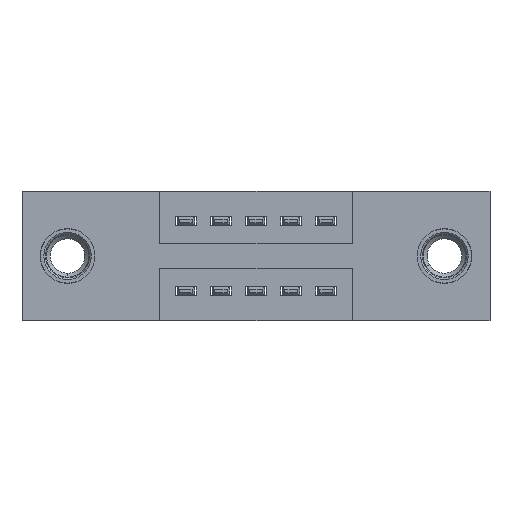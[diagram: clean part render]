
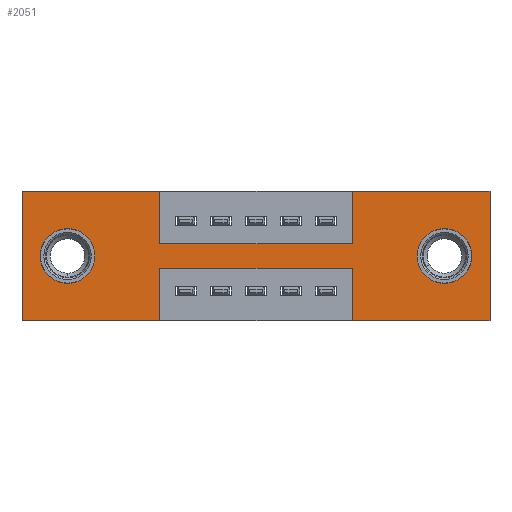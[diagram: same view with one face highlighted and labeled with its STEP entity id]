
A CAD part, front view. The second image highlights one B-rep face of the part: STEP entity #2051.
In plain terms, the highlighted planar face has unit normal (0, -1, 0).
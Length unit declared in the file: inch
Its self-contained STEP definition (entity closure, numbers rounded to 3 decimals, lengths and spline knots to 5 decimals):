
#23 = VECTOR ( 'NONE', #9849, 39.37008 ) ;
#76 = PLANE ( 'NONE',  #353 ) ;
#247 = VERTEX_POINT ( 'NONE', #6953 ) ;
#253 = VERTEX_POINT ( 'NONE', #6856 ) ;
#286 = VECTOR ( 'NONE', #4858, 39.37008 ) ;
#353 = AXIS2_PLACEMENT_3D ( 'NONE', #4833, #5645, #920 ) ;
#389 = CARTESIAN_POINT ( 'NONE',  ( 1.205, 0., -0.263 ) ) ;
#519 = EDGE_CURVE ( 'NONE', #6847, #3783, #5435, .T. ) ;
#687 = CARTESIAN_POINT ( 'NONE',  ( 0., 0., 0. ) ) ;
#796 = VERTEX_POINT ( 'NONE', #8896 ) ;
#920 = DIRECTION ( 'NONE',  ( 0., 0., -1. ) ) ;
#983 = LINE ( 'NONE', #6651, #5181 ) ;
#1029 = DIRECTION ( 'NONE',  ( 0., 1., 0. ) ) ;
#1256 = EDGE_CURVE ( 'NONE', #4282, #253, #4956, .T. ) ;
#1284 = ORIENTED_EDGE ( 'NONE', *, *, #4645, .F. ) ;
#1444 = CARTESIAN_POINT ( 'NONE',  ( 0., 0., 0. ) ) ;
#1523 = ORIENTED_EDGE ( 'NONE', *, *, #8774, .F. ) ;
#1524 = DIRECTION ( 'NONE',  ( 0., 1., 0. ) ) ;
#1586 = VERTEX_POINT ( 'NONE', #7264 ) ;
#1705 = EDGE_CURVE ( 'NONE', #2841, #247, #983, .T. ) ;
#1823 = LINE ( 'NONE', #3899, #7775 ) ;
#1859 = DIRECTION ( 'NONE',  ( -1., 0., 0. ) ) ;
#1946 = DIRECTION ( 'NONE',  ( 0., 0., -1. ) ) ;
#1976 = EDGE_CURVE ( 'NONE', #4321, #1586, #8781, .T. ) ;
#1998 = VERTEX_POINT ( 'NONE', #6342 ) ;
#2031 = LINE ( 'NONE', #8021, #5756 ) ;
#2051 = ADVANCED_FACE ( 'NONE', ( #4059, #5910, #9777 ), #76, .T. ) ;
#2053 = CARTESIAN_POINT ( 'NONE',  ( 0.3925, 0., -0.37 ) ) ;
#2192 = DIRECTION ( 'NONE',  ( 0., 0., 1. ) ) ;
#2251 = ORIENTED_EDGE ( 'NONE', *, *, #3698, .F. ) ;
#2294 = CARTESIAN_POINT ( 'NONE',  ( 0.9425, 0., -0.37 ) ) ;
#2376 = CARTESIAN_POINT ( 'NONE',  ( 0.3925, 0., -0.22 ) ) ;
#2602 = VERTEX_POINT ( 'NONE', #2294 ) ;
#2687 = DIRECTION ( 'NONE',  ( 0., 0., 1. ) ) ;
#2797 = CARTESIAN_POINT ( 'NONE',  ( 0.3925, 0., -0.15 ) ) ;
#2817 = CARTESIAN_POINT ( 'NONE',  ( 0., 0., 0. ) ) ;
#2841 = VERTEX_POINT ( 'NONE', #5771 ) ;
#2936 = DIRECTION ( 'NONE',  ( 0., 1., 0. ) ) ;
#3103 = VECTOR ( 'NONE', #8829, 39.37008 ) ;
#3146 = ORIENTED_EDGE ( 'NONE', *, *, #1256, .T. ) ;
#3198 = DIRECTION ( 'NONE',  ( -1., 0., 0. ) ) ;
#3405 = DIRECTION ( 'NONE',  ( 0., 0., 1. ) ) ;
#3530 = CARTESIAN_POINT ( 'NONE',  ( 0.3925, 0., -0.15 ) ) ;
#3638 = VERTEX_POINT ( 'NONE', #389 ) ;
#3679 = CARTESIAN_POINT ( 'NONE',  ( 0., 0., -0.37 ) ) ;
#3698 = EDGE_CURVE ( 'NONE', #6003, #796, #7973, .T. ) ;
#3783 = VERTEX_POINT ( 'NONE', #3679 ) ;
#3899 = CARTESIAN_POINT ( 'NONE',  ( 0., 0., 0. ) ) ;
#3901 = CARTESIAN_POINT ( 'NONE',  ( 0.13, 0., -0.185 ) ) ;
#3908 = EDGE_CURVE ( 'NONE', #253, #4282, #6335, .T. ) ;
#3953 = CARTESIAN_POINT ( 'NONE',  ( 1.205, 0., -0.107 ) ) ;
#3976 = VERTEX_POINT ( 'NONE', #3953 ) ;
#4059 = FACE_BOUND ( 'NONE', #4944, .T. ) ;
#4075 = CARTESIAN_POINT ( 'NONE',  ( 0.3925, 0., -0.37 ) ) ;
#4282 = VERTEX_POINT ( 'NONE', #5630 ) ;
#4311 = EDGE_CURVE ( 'NONE', #796, #4584, #8286, .T. ) ;
#4321 = VERTEX_POINT ( 'NONE', #6428 ) ;
#4383 = LINE ( 'NONE', #2053, #5729 ) ;
#4426 = DIRECTION ( 'NONE',  ( -1., 0., 0. ) ) ;
#4584 = VERTEX_POINT ( 'NONE', #2797 ) ;
#4645 = EDGE_CURVE ( 'NONE', #1586, #6847, #4383, .T. ) ;
#4709 = DIRECTION ( 'NONE',  ( 1., 0., 0. ) ) ;
#4761 = ORIENTED_EDGE ( 'NONE', *, *, #9140, .T. ) ;
#4783 = EDGE_LOOP ( 'NONE', ( #3146, #5253 ) ) ;
#4833 = CARTESIAN_POINT ( 'NONE',  ( 0., 0., -0.37 ) ) ;
#4858 = DIRECTION ( 'NONE',  ( 0., 0., -1. ) ) ;
#4890 = EDGE_LOOP ( 'NONE', ( #1284, #5493, #7518, #1523, #5738, #5987, #9840, #6217, #8183, #2251, #6452, #8404 ) ) ;
#4944 = EDGE_LOOP ( 'NONE', ( #4761, #6802 ) ) ;
#4956 = CIRCLE ( 'NONE', #5198, 0.078 ) ;
#5164 = LINE ( 'NONE', #6000, #9336 ) ;
#5176 = AXIS2_PLACEMENT_3D ( 'NONE', #5752, #1029, #6513 ) ;
#5181 = VECTOR ( 'NONE', #1946, 39.37008 ) ;
#5198 = AXIS2_PLACEMENT_3D ( 'NONE', #3901, #5206, #2687 ) ;
#5206 = DIRECTION ( 'NONE',  ( 0., 1., 0. ) ) ;
#5207 = LINE ( 'NONE', #3530, #3103 ) ;
#5253 = ORIENTED_EDGE ( 'NONE', *, *, #3908, .T. ) ;
#5435 = LINE ( 'NONE', #8944, #8912 ) ;
#5493 = ORIENTED_EDGE ( 'NONE', *, *, #1976, .F. ) ;
#5630 = CARTESIAN_POINT ( 'NONE',  ( 0.13, 0., -0.107 ) ) ;
#5643 = CIRCLE ( 'NONE', #5176, 0.078 ) ;
#5645 = DIRECTION ( 'NONE',  ( 0., -1., 0. ) ) ;
#5729 = VECTOR ( 'NONE', #6757, 39.37008 ) ;
#5738 = ORIENTED_EDGE ( 'NONE', *, *, #1705, .F. ) ;
#5752 = CARTESIAN_POINT ( 'NONE',  ( 1.205, 0., -0.185 ) ) ;
#5756 = VECTOR ( 'NONE', #3405, 39.37008 ) ;
#5771 = CARTESIAN_POINT ( 'NONE',  ( 1.335, 0., 0. ) ) ;
#5910 = FACE_BOUND ( 'NONE', #4783, .T. ) ;
#5987 = ORIENTED_EDGE ( 'NONE', *, *, #8471, .F. ) ;
#5998 = VECTOR ( 'NONE', #7487, 39.37008 ) ;
#6000 = CARTESIAN_POINT ( 'NONE',  ( 0., 0., -0.37 ) ) ;
#6003 = VERTEX_POINT ( 'NONE', #1444 ) ;
#6142 = CARTESIAN_POINT ( 'NONE',  ( 0.9425, 0., 0. ) ) ;
#6217 = ORIENTED_EDGE ( 'NONE', *, *, #6390, .F. ) ;
#6248 = CARTESIAN_POINT ( 'NONE',  ( 0.13, 0., -0.185 ) ) ;
#6335 = CIRCLE ( 'NONE', #8044, 0.078 ) ;
#6342 = CARTESIAN_POINT ( 'NONE',  ( 0.9425, 0., -0.15 ) ) ;
#6390 = EDGE_CURVE ( 'NONE', #4584, #1998, #5207, .T. ) ;
#6428 = CARTESIAN_POINT ( 'NONE',  ( 0.9425, 0., -0.22 ) ) ;
#6452 = ORIENTED_EDGE ( 'NONE', *, *, #9507, .F. ) ;
#6513 = DIRECTION ( 'NONE',  ( 0., 0., -1. ) ) ;
#6617 = VECTOR ( 'NONE', #3198, 39.37008 ) ;
#6651 = CARTESIAN_POINT ( 'NONE',  ( 1.335, 0., 0. ) ) ;
#6757 = DIRECTION ( 'NONE',  ( 0., 0., -1. ) ) ;
#6802 = ORIENTED_EDGE ( 'NONE', *, *, #8307, .T. ) ;
#6847 = VERTEX_POINT ( 'NONE', #4075 ) ;
#6856 = CARTESIAN_POINT ( 'NONE',  ( 0.13, 0., -0.263 ) ) ;
#6953 = CARTESIAN_POINT ( 'NONE',  ( 1.335, 0., -0.37 ) ) ;
#6971 = LINE ( 'NONE', #6142, #8673 ) ;
#7003 = DIRECTION ( 'NONE',  ( 0., 0., 1. ) ) ;
#7264 = CARTESIAN_POINT ( 'NONE',  ( 0.3925, 0., -0.22 ) ) ;
#7297 = AXIS2_PLACEMENT_3D ( 'NONE', #7596, #2936, #8292 ) ;
#7487 = DIRECTION ( 'NONE',  ( 1., 0., 0. ) ) ;
#7518 = ORIENTED_EDGE ( 'NONE', *, *, #9788, .F. ) ;
#7596 = CARTESIAN_POINT ( 'NONE',  ( 1.205, 0., -0.185 ) ) ;
#7775 = VECTOR ( 'NONE', #4709, 39.37008 ) ;
#7973 = LINE ( 'NONE', #2817, #5998 ) ;
#8021 = CARTESIAN_POINT ( 'NONE',  ( 0.9425, 0., -0.37 ) ) ;
#8044 = AXIS2_PLACEMENT_3D ( 'NONE', #6248, #1524, #7003 ) ;
#8183 = ORIENTED_EDGE ( 'NONE', *, *, #4311, .F. ) ;
#8286 = LINE ( 'NONE', #9328, #286 ) ;
#8292 = DIRECTION ( 'NONE',  ( 0., 0., -1. ) ) ;
#8307 = EDGE_CURVE ( 'NONE', #3638, #3976, #9346, .T. ) ;
#8309 = LINE ( 'NONE', #687, #23 ) ;
#8366 = EDGE_CURVE ( 'NONE', #1998, #8954, #6971, .T. ) ;
#8404 = ORIENTED_EDGE ( 'NONE', *, *, #519, .F. ) ;
#8409 = CARTESIAN_POINT ( 'NONE',  ( 0.9425, 0., 0. ) ) ;
#8471 = EDGE_CURVE ( 'NONE', #8954, #2841, #1823, .T. ) ;
#8673 = VECTOR ( 'NONE', #2192, 39.37008 ) ;
#8774 = EDGE_CURVE ( 'NONE', #247, #2602, #5164, .T. ) ;
#8781 = LINE ( 'NONE', #2376, #6617 ) ;
#8829 = DIRECTION ( 'NONE',  ( 1., 0., 0. ) ) ;
#8896 = CARTESIAN_POINT ( 'NONE',  ( 0.3925, 0., 0. ) ) ;
#8912 = VECTOR ( 'NONE', #1859, 39.37008 ) ;
#8944 = CARTESIAN_POINT ( 'NONE',  ( 0., 0., -0.37 ) ) ;
#8954 = VERTEX_POINT ( 'NONE', #8409 ) ;
#9140 = EDGE_CURVE ( 'NONE', #3976, #3638, #5643, .T. ) ;
#9328 = CARTESIAN_POINT ( 'NONE',  ( 0.3925, 0., 0. ) ) ;
#9336 = VECTOR ( 'NONE', #4426, 39.37008 ) ;
#9346 = CIRCLE ( 'NONE', #7297, 0.078 ) ;
#9507 = EDGE_CURVE ( 'NONE', #3783, #6003, #8309, .T. ) ;
#9777 = FACE_OUTER_BOUND ( 'NONE', #4890, .T. ) ;
#9788 = EDGE_CURVE ( 'NONE', #2602, #4321, #2031, .T. ) ;
#9840 = ORIENTED_EDGE ( 'NONE', *, *, #8366, .F. ) ;
#9849 = DIRECTION ( 'NONE',  ( 0., 0., 1. ) ) ;
